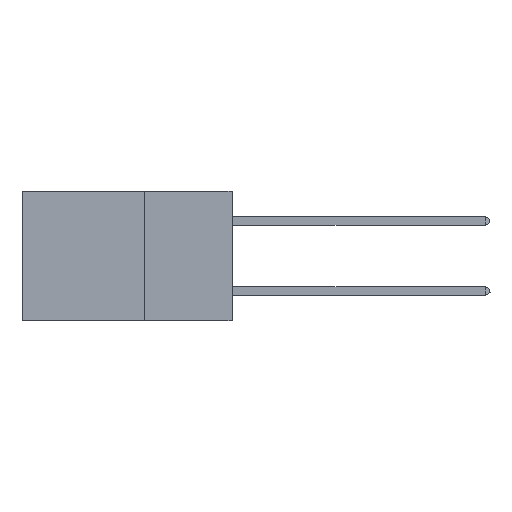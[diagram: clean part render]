
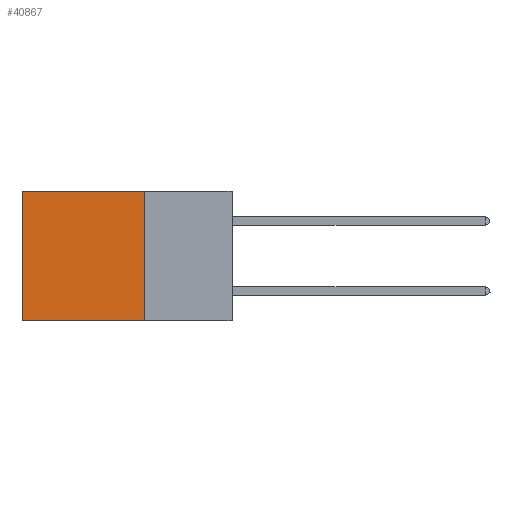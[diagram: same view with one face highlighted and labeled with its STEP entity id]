
A CAD part, left-side view. The second image highlights one B-rep face of the part: STEP entity #40867.
In plain terms, the highlighted planar face has unit normal (-1, 0, 0).
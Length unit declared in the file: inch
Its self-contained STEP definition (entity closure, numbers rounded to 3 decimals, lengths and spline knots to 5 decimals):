
#740 = CARTESIAN_POINT ( 'NONE',  ( 0.2875, 0.6, 0. ) ) ;
#2115 = VECTOR ( 'NONE', #18663, 39.37008 ) ;
#2900 = CARTESIAN_POINT ( 'NONE',  ( 0.2875, 0.6, -0.37 ) ) ;
#3584 = ORIENTED_EDGE ( 'NONE', *, *, #35306, .T. ) ;
#3633 = CARTESIAN_POINT ( 'NONE',  ( 0.2875, 0.25, 0. ) ) ;
#6664 = DIRECTION ( 'NONE',  ( 0., 0., -1. ) ) ;
#10230 = EDGE_LOOP ( 'NONE', ( #3584, #25219, #34835, #14895 ) ) ;
#10759 = VERTEX_POINT ( 'NONE', #2900 ) ;
#11056 = LINE ( 'NONE', #31272, #39617 ) ;
#11442 = PLANE ( 'NONE',  #25343 ) ;
#13362 = LINE ( 'NONE', #16202, #2115 ) ;
#14895 = ORIENTED_EDGE ( 'NONE', *, *, #19115, .T. ) ;
#16202 = CARTESIAN_POINT ( 'NONE',  ( 0.2875, 0.25, -0.37 ) ) ;
#18663 = DIRECTION ( 'NONE',  ( 0., 1., 0. ) ) ;
#19115 = EDGE_CURVE ( 'NONE', #33009, #28788, #19691, .T. ) ;
#19691 = LINE ( 'NONE', #22315, #36104 ) ;
#20151 = LINE ( 'NONE', #29074, #31517 ) ;
#21860 = CARTESIAN_POINT ( 'NONE',  ( 0.2875, 0.25, 0. ) ) ;
#22315 = CARTESIAN_POINT ( 'NONE',  ( 0.2875, 0.25, 0. ) ) ;
#24088 = DIRECTION ( 'NONE',  ( 0., 0., -1. ) ) ;
#24698 = DIRECTION ( 'NONE',  ( 1., 0., 0. ) ) ;
#25219 = ORIENTED_EDGE ( 'NONE', *, *, #31540, .F. ) ;
#25343 = AXIS2_PLACEMENT_3D ( 'NONE', #21860, #24698, #37949 ) ;
#27155 = VERTEX_POINT ( 'NONE', #28802 ) ;
#28788 = VERTEX_POINT ( 'NONE', #740 ) ;
#28802 = CARTESIAN_POINT ( 'NONE',  ( 0.2875, 0.25, -0.37 ) ) ;
#29074 = CARTESIAN_POINT ( 'NONE',  ( 0.2875, 0.6, 0. ) ) ;
#31272 = CARTESIAN_POINT ( 'NONE',  ( 0.2875, 0.25, 0. ) ) ;
#31359 = EDGE_CURVE ( 'NONE', #33009, #27155, #11056, .T. ) ;
#31517 = VECTOR ( 'NONE', #6664, 39.37008 ) ;
#31540 = EDGE_CURVE ( 'NONE', #27155, #10759, #13362, .T. ) ;
#33009 = VERTEX_POINT ( 'NONE', #3633 ) ;
#34258 = FACE_OUTER_BOUND ( 'NONE', #10230, .T. ) ;
#34835 = ORIENTED_EDGE ( 'NONE', *, *, #31359, .F. ) ;
#35306 = EDGE_CURVE ( 'NONE', #28788, #10759, #20151, .T. ) ;
#36104 = VECTOR ( 'NONE', #42744, 39.37008 ) ;
#37949 = DIRECTION ( 'NONE',  ( 0., 0., -1. ) ) ;
#39617 = VECTOR ( 'NONE', #24088, 39.37008 ) ;
#40867 = ADVANCED_FACE ( 'NONE', ( #34258 ), #11442, .F. ) ;
#42744 = DIRECTION ( 'NONE',  ( 0., 1., 0. ) ) ;
